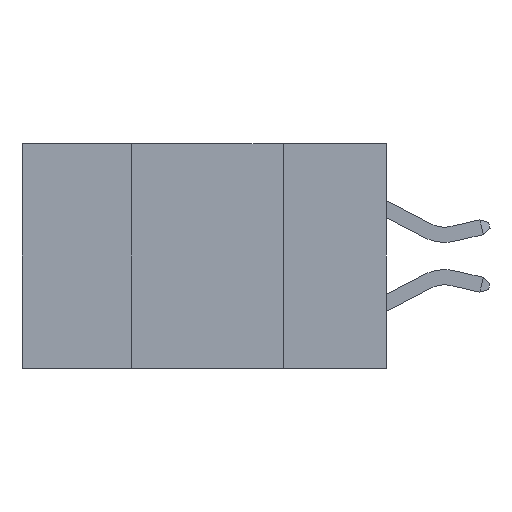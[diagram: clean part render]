
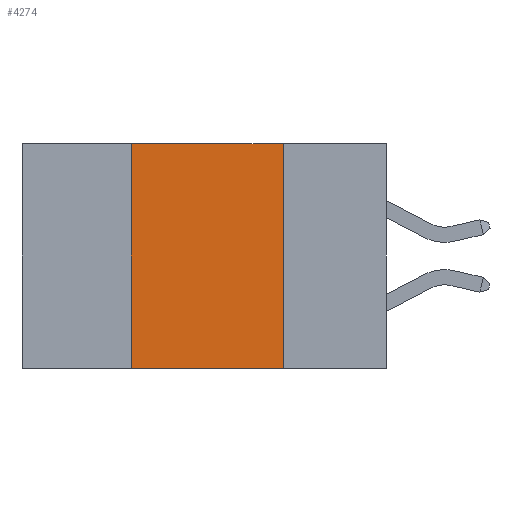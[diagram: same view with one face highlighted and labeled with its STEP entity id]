
A CAD part, left-side view. The second image highlights one B-rep face of the part: STEP entity #4274.
In plain terms, the highlighted planar face has unit normal (-1, 0, 0).
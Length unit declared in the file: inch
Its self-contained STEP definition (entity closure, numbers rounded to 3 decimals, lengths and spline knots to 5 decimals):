
#293 = VECTOR ( 'NONE', #594, 39.37008 ) ;
#454 = CARTESIAN_POINT ( 'NONE',  ( 0., 0.6, 0. ) ) ;
#594 = DIRECTION ( 'NONE',  ( 0., -1., 0. ) ) ;
#2565 = VERTEX_POINT ( 'NONE', #10069 ) ;
#3023 = CARTESIAN_POINT ( 'NONE',  ( 0., 0.17, -0.37 ) ) ;
#3375 = VERTEX_POINT ( 'NONE', #9625 ) ;
#3411 = ORIENTED_EDGE ( 'NONE', *, *, #4137, .F. ) ;
#3438 = ORIENTED_EDGE ( 'NONE', *, *, #4051, .F. ) ;
#3534 = EDGE_CURVE ( 'NONE', #9645, #2565, #4373, .T. ) ;
#3726 = ORIENTED_EDGE ( 'NONE', *, *, #3534, .F. ) ;
#4003 = EDGE_CURVE ( 'NONE', #3375, #5077, #7298, .T. ) ;
#4051 = EDGE_CURVE ( 'NONE', #3375, #9645, #5253, .T. ) ;
#4135 = DIRECTION ( 'NONE',  ( 0., 0., -1. ) ) ;
#4137 = EDGE_CURVE ( 'NONE', #2565, #5077, #5374, .T. ) ;
#4274 = ADVANCED_FACE ( 'NONE', ( #9704 ), #4302, .F. ) ;
#4302 = PLANE ( 'NONE',  #7835 ) ;
#4373 = LINE ( 'NONE', #454, #293 ) ;
#4746 = VECTOR ( 'NONE', #8567, 39.37008 ) ;
#4945 = CARTESIAN_POINT ( 'NONE',  ( 0., 0.6, 0. ) ) ;
#5077 = VERTEX_POINT ( 'NONE', #3023 ) ;
#5186 = EDGE_LOOP ( 'NONE', ( #3411, #3726, #3438, #8329 ) ) ;
#5253 = LINE ( 'NONE', #9524, #4746 ) ;
#5374 = LINE ( 'NONE', #7816, #6091 ) ;
#6091 = VECTOR ( 'NONE', #7757, 39.37008 ) ;
#7115 = CARTESIAN_POINT ( 'NONE',  ( 0., 0.42, 0. ) ) ;
#7298 = LINE ( 'NONE', #7476, #9263 ) ;
#7399 = DIRECTION ( 'NONE',  ( 0., -1., 0. ) ) ;
#7476 = CARTESIAN_POINT ( 'NONE',  ( 0., 0.6, -0.37 ) ) ;
#7757 = DIRECTION ( 'NONE',  ( 0., 0., -1. ) ) ;
#7816 = CARTESIAN_POINT ( 'NONE',  ( 0., 0.17, 0. ) ) ;
#7835 = AXIS2_PLACEMENT_3D ( 'NONE', #4945, #9565, #4135 ) ;
#8329 = ORIENTED_EDGE ( 'NONE', *, *, #4003, .T. ) ;
#8567 = DIRECTION ( 'NONE',  ( 0., 0., 1. ) ) ;
#9263 = VECTOR ( 'NONE', #7399, 39.37008 ) ;
#9524 = CARTESIAN_POINT ( 'NONE',  ( 0., 0.42, 0. ) ) ;
#9565 = DIRECTION ( 'NONE',  ( 1., 0., 0. ) ) ;
#9625 = CARTESIAN_POINT ( 'NONE',  ( 0., 0.42, -0.37 ) ) ;
#9645 = VERTEX_POINT ( 'NONE', #7115 ) ;
#9704 = FACE_OUTER_BOUND ( 'NONE', #5186, .T. ) ;
#10069 = CARTESIAN_POINT ( 'NONE',  ( 0., 0.17, 0. ) ) ;
